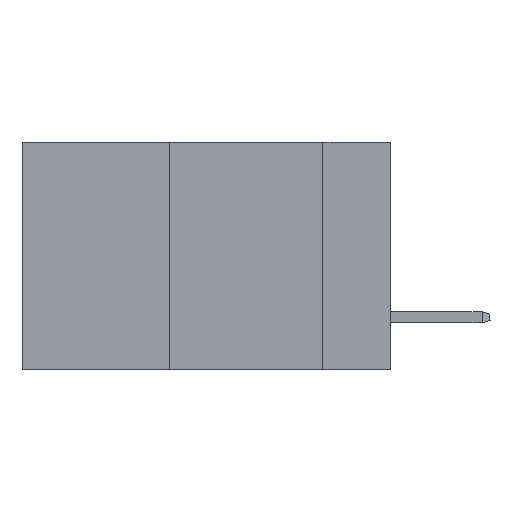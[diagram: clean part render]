
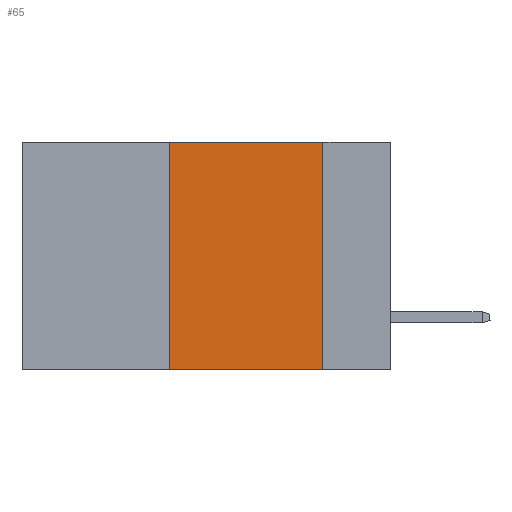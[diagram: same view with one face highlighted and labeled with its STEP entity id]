
A CAD part, left-side view. The second image highlights one B-rep face of the part: STEP entity #65.
In plain terms, the highlighted planar face has unit normal (-1, 0, 0).
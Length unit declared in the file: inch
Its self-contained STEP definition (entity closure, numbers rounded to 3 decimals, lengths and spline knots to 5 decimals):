
#65 = ADVANCED_FACE ( 'NONE', ( #18063 ), #17564, .F. ) ;
#1210 = DIRECTION ( 'NONE',  ( 0., 0., -1. ) ) ;
#1233 = VERTEX_POINT ( 'NONE', #16779 ) ;
#2190 = CARTESIAN_POINT ( 'NONE',  ( 0., 0.36, 0. ) ) ;
#2362 = CARTESIAN_POINT ( 'NONE',  ( 0., 0.6, -0.37 ) ) ;
#2585 = EDGE_CURVE ( 'NONE', #3193, #1233, #16707, .T. ) ;
#3193 = VERTEX_POINT ( 'NONE', #3822 ) ;
#3220 = AXIS2_PLACEMENT_3D ( 'NONE', #14720, #15888, #6382 ) ;
#3822 = CARTESIAN_POINT ( 'NONE',  ( 0., 0.36, -0.37 ) ) ;
#3958 = EDGE_CURVE ( 'NONE', #3193, #12180, #15329, .T. ) ;
#4174 = VECTOR ( 'NONE', #7876, 39.37008 ) ;
#5374 = LINE ( 'NONE', #17767, #6942 ) ;
#6382 = DIRECTION ( 'NONE',  ( 0., 0., -1. ) ) ;
#6942 = VECTOR ( 'NONE', #1210, 39.37008 ) ;
#7876 = DIRECTION ( 'NONE',  ( 0., 0., 1. ) ) ;
#7927 = ORIENTED_EDGE ( 'NONE', *, *, #12202, .F. ) ;
#8125 = CARTESIAN_POINT ( 'NONE',  ( 0., 0.36, 0. ) ) ;
#9271 = ORIENTED_EDGE ( 'NONE', *, *, #9377, .F. ) ;
#9377 = EDGE_CURVE ( 'NONE', #13105, #1233, #5374, .T. ) ;
#9462 = DIRECTION ( 'NONE',  ( 0., -1., 0. ) ) ;
#11828 = ORIENTED_EDGE ( 'NONE', *, *, #2585, .T. ) ;
#12180 = VERTEX_POINT ( 'NONE', #2190 ) ;
#12202 = EDGE_CURVE ( 'NONE', #12180, #13105, #14015, .T. ) ;
#12720 = EDGE_LOOP ( 'NONE', ( #9271, #7927, #14952, #11828 ) ) ;
#13105 = VERTEX_POINT ( 'NONE', #15748 ) ;
#13186 = CARTESIAN_POINT ( 'NONE',  ( 0., 0.6, 0. ) ) ;
#13415 = DIRECTION ( 'NONE',  ( 0., -1., 0. ) ) ;
#14015 = LINE ( 'NONE', #13186, #16659 ) ;
#14720 = CARTESIAN_POINT ( 'NONE',  ( 0., 0.6, 0. ) ) ;
#14952 = ORIENTED_EDGE ( 'NONE', *, *, #3958, .F. ) ;
#15329 = LINE ( 'NONE', #8125, #4174 ) ;
#15748 = CARTESIAN_POINT ( 'NONE',  ( 0., 0.11, 0. ) ) ;
#15888 = DIRECTION ( 'NONE',  ( 1., 0., 0. ) ) ;
#16255 = VECTOR ( 'NONE', #9462, 39.37008 ) ;
#16659 = VECTOR ( 'NONE', #13415, 39.37008 ) ;
#16707 = LINE ( 'NONE', #2362, #16255 ) ;
#16779 = CARTESIAN_POINT ( 'NONE',  ( 0., 0.11, -0.37 ) ) ;
#17564 = PLANE ( 'NONE',  #3220 ) ;
#17767 = CARTESIAN_POINT ( 'NONE',  ( 0., 0.11, 0. ) ) ;
#18063 = FACE_OUTER_BOUND ( 'NONE', #12720, .T. ) ;
